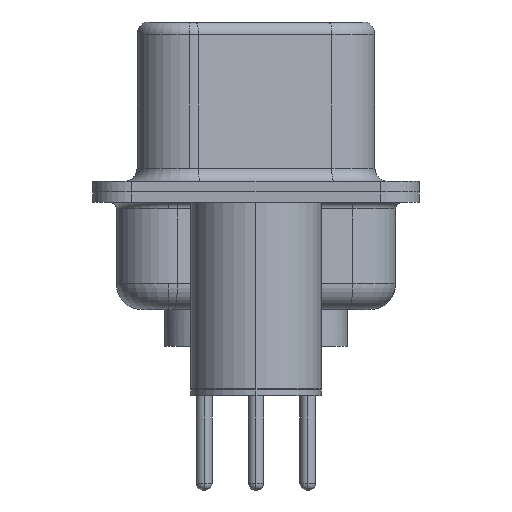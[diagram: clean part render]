
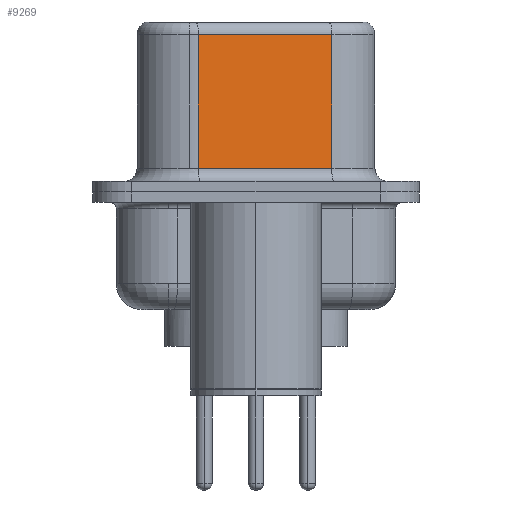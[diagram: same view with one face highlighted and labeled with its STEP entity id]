
A CAD part, left-side view. The second image highlights one B-rep face of the part: STEP entity #9269.
In plain terms, the highlighted planar face has unit normal (-0.985, -0.174, 0).
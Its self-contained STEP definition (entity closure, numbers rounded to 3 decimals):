
#498 = EDGE_LOOP ( 'NONE', ( #1344, #18173, #9099, #24147 ) ) ;
#1319 = DIRECTION ( 'NONE',  ( 0., 0., -1. ) ) ;
#1344 = ORIENTED_EDGE ( 'NONE', *, *, #19699, .F. ) ;
#2995 = FACE_OUTER_BOUND ( 'NONE', #498, .T. ) ;
#4737 = LINE ( 'NONE', #14646, #26347 ) ;
#5300 = EDGE_CURVE ( 'NONE', #22731, #17441, #10807, .T. ) ;
#5888 = CARTESIAN_POINT ( 'NONE',  ( 4.58, -2.897, 6.52 ) ) ;
#7774 = EDGE_CURVE ( 'NONE', #10161, #12969, #4737, .T. ) ;
#8032 = DIRECTION ( 'NONE',  ( -0.174, 0.985, 0. ) ) ;
#8175 = CARTESIAN_POINT ( 'NONE',  ( 4.58, -2.897, 0.9 ) ) ;
#9099 = ORIENTED_EDGE ( 'NONE', *, *, #18896, .T. ) ;
#9269 = ADVANCED_FACE ( 'NONE', ( #2995 ), #14268, .F. ) ;
#9541 = VECTOR ( 'NONE', #1319, 1000. ) ;
#10161 = VERTEX_POINT ( 'NONE', #11094 ) ;
#10310 = CARTESIAN_POINT ( 'NONE',  ( 4.58, -2.897, 6.52 ) ) ;
#10510 = VECTOR ( 'NONE', #24891, 1000. ) ;
#10527 = VECTOR ( 'NONE', #11825, 1000. ) ;
#10807 = LINE ( 'NONE', #11954, #10527 ) ;
#11094 = CARTESIAN_POINT ( 'NONE',  ( 4.58, -2.897, 6.02 ) ) ;
#11825 = DIRECTION ( 'NONE',  ( 0.174, -0.985, 0. ) ) ;
#11954 = CARTESIAN_POINT ( 'NONE',  ( 4.58, -2.897, 0.9 ) ) ;
#12969 = VERTEX_POINT ( 'NONE', #23689 ) ;
#14268 = PLANE ( 'NONE',  #19827 ) ;
#14646 = CARTESIAN_POINT ( 'NONE',  ( 4.58, -2.897, 6.02 ) ) ;
#15581 = DIRECTION ( 'NONE',  ( -0.174, 0.985, 0. ) ) ;
#17441 = VERTEX_POINT ( 'NONE', #8175 ) ;
#18119 = CARTESIAN_POINT ( 'NONE',  ( 3.68, 2.203, 6.52 ) ) ;
#18173 = ORIENTED_EDGE ( 'NONE', *, *, #7774, .T. ) ;
#18215 = CARTESIAN_POINT ( 'NONE',  ( 3.68, 2.203, 0.9 ) ) ;
#18896 = EDGE_CURVE ( 'NONE', #12969, #22731, #20677, .T. ) ;
#19699 = EDGE_CURVE ( 'NONE', #10161, #17441, #21597, .T. ) ;
#19827 = AXIS2_PLACEMENT_3D ( 'NONE', #5888, #20550, #8032 ) ;
#20550 = DIRECTION ( 'NONE',  ( 0.985, 0.174, 0. ) ) ;
#20677 = LINE ( 'NONE', #18119, #9541 ) ;
#21597 = LINE ( 'NONE', #10310, #10510 ) ;
#22731 = VERTEX_POINT ( 'NONE', #18215 ) ;
#23689 = CARTESIAN_POINT ( 'NONE',  ( 3.68, 2.203, 6.02 ) ) ;
#24147 = ORIENTED_EDGE ( 'NONE', *, *, #5300, .T. ) ;
#24891 = DIRECTION ( 'NONE',  ( 0., 0., -1. ) ) ;
#26347 = VECTOR ( 'NONE', #15581, 1000. ) ;
